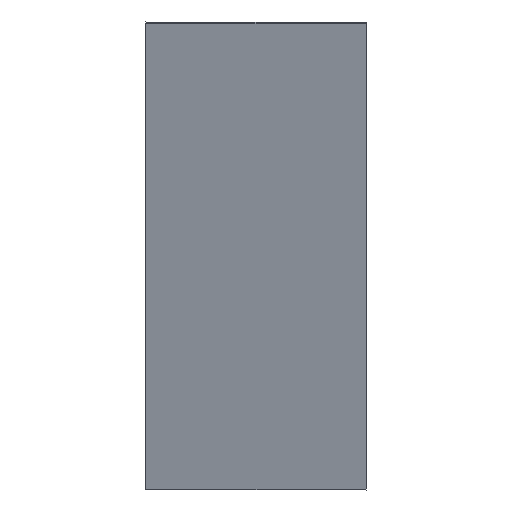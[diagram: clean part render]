
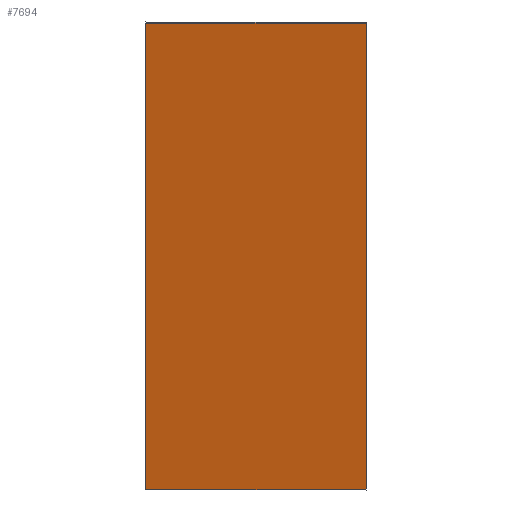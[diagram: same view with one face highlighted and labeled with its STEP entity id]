
A CAD part, front view. The second image highlights one B-rep face of the part: STEP entity #7694.
In plain terms, the highlighted planar face has unit normal (0, -0.97, -0.241).
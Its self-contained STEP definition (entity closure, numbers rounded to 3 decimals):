
#929=FACE_OUTER_BOUND('',#1410,.T.);
#1410=EDGE_LOOP('',(#5291,#5292,#5293,#5294));
#1973=LINE('',#12459,#2558);
#1976=LINE('',#12465,#2561);
#1979=LINE('',#12471,#2564);
#1982=LINE('',#12475,#2567);
#2558=VECTOR('',#9185,10.);
#2561=VECTOR('',#9190,10.);
#2564=VECTOR('',#9195,10.);
#2567=VECTOR('',#9200,10.);
#3262=VERTEX_POINT('',#12456);
#3263=VERTEX_POINT('',#12458);
#3265=VERTEX_POINT('',#12464);
#3267=VERTEX_POINT('',#12470);
#4031=EDGE_CURVE('',#3263,#3262,#1973,.T.);
#4034=EDGE_CURVE('',#3265,#3263,#1976,.T.);
#4037=EDGE_CURVE('',#3267,#3265,#1979,.T.);
#4040=EDGE_CURVE('',#3262,#3267,#1982,.T.);
#5291=ORIENTED_EDGE('',*,*,#4040,.T.);
#5292=ORIENTED_EDGE('',*,*,#4037,.T.);
#5293=ORIENTED_EDGE('',*,*,#4034,.T.);
#5294=ORIENTED_EDGE('',*,*,#4031,.T.);
#7512=PLANE('',#8234);
#7694=ADVANCED_FACE('',(#929),#7512,.T.);
#8234=AXIS2_PLACEMENT_3D('',#12476,#9201,#9202);
#9185=DIRECTION('',(0.,-0.241,0.97));
#9190=DIRECTION('',(1.,0.,0.));
#9195=DIRECTION('',(0.,0.241,-0.97));
#9200=DIRECTION('',(-1.,0.,0.));
#9201=DIRECTION('center_axis',(0.,-0.97,-0.241));
#9202=DIRECTION('ref_axis',(0.,0.241,-0.97));
#12456=CARTESIAN_POINT('',(23.996,-119.903,36.563));
#12458=CARTESIAN_POINT('',(23.996,-94.846,-64.147));
#12459=CARTESIAN_POINT('',(23.996,-94.846,-64.147));
#12464=CARTESIAN_POINT('',(-23.674,-94.846,-64.147));
#12465=CARTESIAN_POINT('',(-23.674,-94.846,-64.147));
#12470=CARTESIAN_POINT('',(-23.674,-119.903,36.563));
#12471=CARTESIAN_POINT('',(-23.674,-119.903,36.563));
#12475=CARTESIAN_POINT('',(23.996,-119.903,36.563));
#12476=CARTESIAN_POINT('Origin',(0.161,-107.374,-13.792));
